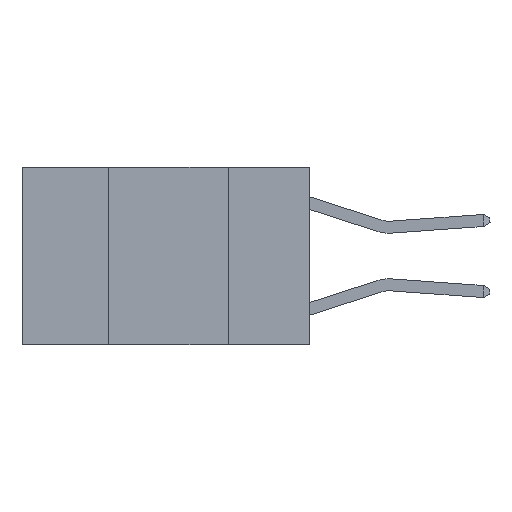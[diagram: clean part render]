
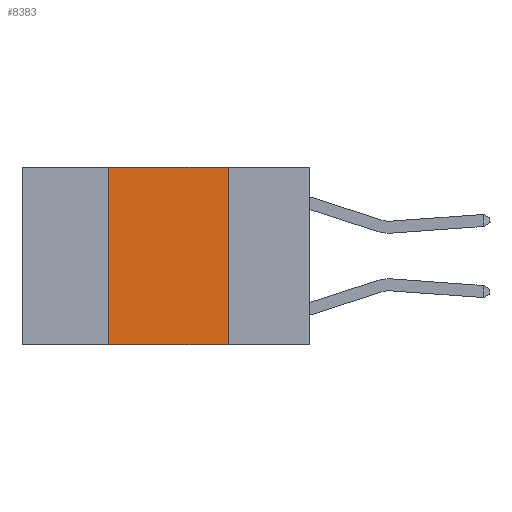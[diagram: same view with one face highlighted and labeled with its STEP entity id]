
A CAD part, left-side view. The second image highlights one B-rep face of the part: STEP entity #8383.
In plain terms, the highlighted planar face has unit normal (-1, 0, 0).
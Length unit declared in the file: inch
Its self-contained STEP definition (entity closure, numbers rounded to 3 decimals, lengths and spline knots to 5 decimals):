
#887 = LINE ( 'NONE', #4167, #9395 ) ;
#1093 = AXIS2_PLACEMENT_3D ( 'NONE', #3872, #7061, #6990 ) ;
#1181 = EDGE_CURVE ( 'NONE', #8655, #11739, #887, .T. ) ;
#1227 = DIRECTION ( 'NONE',  ( 0., -1., 0. ) ) ;
#1964 = PLANE ( 'NONE',  #1093 ) ;
#2117 = EDGE_CURVE ( 'NONE', #8655, #4214, #13149, .T. ) ;
#2419 = VECTOR ( 'NONE', #6268, 39.37008 ) ;
#2774 = EDGE_CURVE ( 'NONE', #4214, #4876, #6324, .T. ) ;
#3245 = CARTESIAN_POINT ( 'NONE',  ( 0., 0.17, -0.37 ) ) ;
#3387 = VECTOR ( 'NONE', #10873, 39.37008 ) ;
#3739 = CARTESIAN_POINT ( 'NONE',  ( 0., 0.42, 0. ) ) ;
#3860 = ORIENTED_EDGE ( 'NONE', *, *, #2774, .F. ) ;
#3870 = VECTOR ( 'NONE', #1227, 39.37008 ) ;
#3872 = CARTESIAN_POINT ( 'NONE',  ( 0., 0.6, 0. ) ) ;
#4167 = CARTESIAN_POINT ( 'NONE',  ( 0., 0.6, -0.37 ) ) ;
#4189 = CARTESIAN_POINT ( 'NONE',  ( 0., 0.6, 0. ) ) ;
#4191 = CARTESIAN_POINT ( 'NONE',  ( 0., 0.42, 0. ) ) ;
#4214 = VERTEX_POINT ( 'NONE', #4191 ) ;
#4426 = LINE ( 'NONE', #12663, #2419 ) ;
#4799 = FACE_OUTER_BOUND ( 'NONE', #8189, .T. ) ;
#4876 = VERTEX_POINT ( 'NONE', #12149 ) ;
#5596 = CARTESIAN_POINT ( 'NONE',  ( 0., 0.42, -0.37 ) ) ;
#5994 = ORIENTED_EDGE ( 'NONE', *, *, #9072, .F. ) ;
#6268 = DIRECTION ( 'NONE',  ( 0., 0., -1. ) ) ;
#6324 = LINE ( 'NONE', #4189, #3870 ) ;
#6990 = DIRECTION ( 'NONE',  ( 0., 0., -1. ) ) ;
#7061 = DIRECTION ( 'NONE',  ( 1., 0., 0. ) ) ;
#7364 = ORIENTED_EDGE ( 'NONE', *, *, #1181, .T. ) ;
#8189 = EDGE_LOOP ( 'NONE', ( #5994, #3860, #13549, #7364 ) ) ;
#8383 = ADVANCED_FACE ( 'NONE', ( #4799 ), #1964, .F. ) ;
#8655 = VERTEX_POINT ( 'NONE', #5596 ) ;
#9072 = EDGE_CURVE ( 'NONE', #4876, #11739, #4426, .T. ) ;
#9395 = VECTOR ( 'NONE', #9532, 39.37008 ) ;
#9532 = DIRECTION ( 'NONE',  ( 0., -1., 0. ) ) ;
#10873 = DIRECTION ( 'NONE',  ( 0., 0., 1. ) ) ;
#11739 = VERTEX_POINT ( 'NONE', #3245 ) ;
#12149 = CARTESIAN_POINT ( 'NONE',  ( 0., 0.17, 0. ) ) ;
#12663 = CARTESIAN_POINT ( 'NONE',  ( 0., 0.17, 0. ) ) ;
#13149 = LINE ( 'NONE', #3739, #3387 ) ;
#13549 = ORIENTED_EDGE ( 'NONE', *, *, #2117, .F. ) ;
